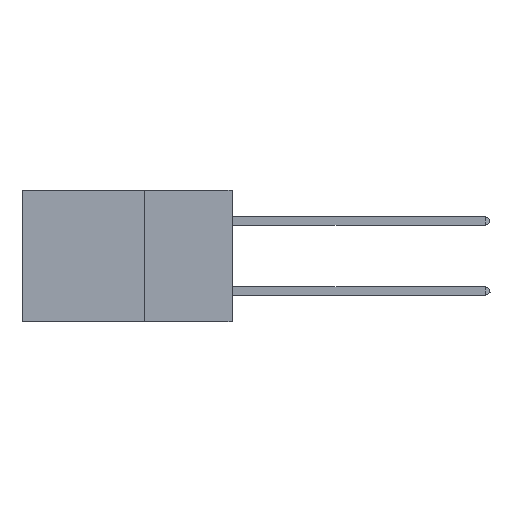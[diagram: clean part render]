
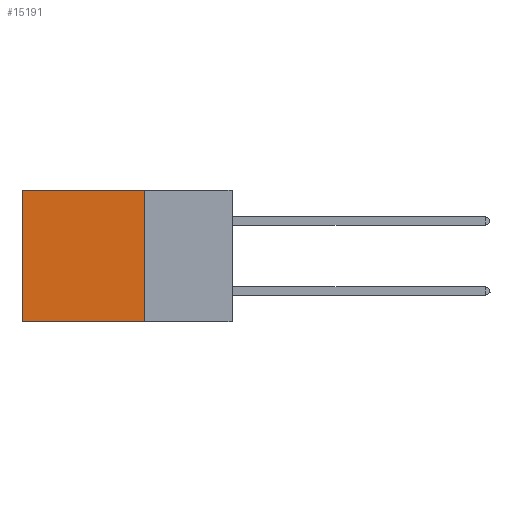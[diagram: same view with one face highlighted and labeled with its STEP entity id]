
A CAD part, left-side view. The second image highlights one B-rep face of the part: STEP entity #15191.
In plain terms, the highlighted planar face has unit normal (-1, 0, 0).
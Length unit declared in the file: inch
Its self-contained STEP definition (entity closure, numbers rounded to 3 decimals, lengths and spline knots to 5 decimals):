
#776 = CARTESIAN_POINT ( 'NONE',  ( 0.2875, 0.25, -0.375 ) ) ;
#837 = EDGE_CURVE ( 'NONE', #12370, #7916, #6039, .T. ) ;
#1363 = LINE ( 'NONE', #6219, #5033 ) ;
#2086 = VERTEX_POINT ( 'NONE', #9191 ) ;
#2201 = VERTEX_POINT ( 'NONE', #2952 ) ;
#2498 = DIRECTION ( 'NONE',  ( 0., 1., 0. ) ) ;
#2951 = AXIS2_PLACEMENT_3D ( 'NONE', #776, #13482, #11012 ) ;
#2952 = CARTESIAN_POINT ( 'NONE',  ( 0.2875, 0.25, -0.375 ) ) ;
#3482 = ORIENTED_EDGE ( 'NONE', *, *, #11682, .T. ) ;
#4158 = DIRECTION ( 'NONE',  ( 0., 1., 0. ) ) ;
#4168 = CARTESIAN_POINT ( 'NONE',  ( 0.2875, 0.25, 0. ) ) ;
#4285 = VECTOR ( 'NONE', #5078, 39.37008 ) ;
#4641 = EDGE_CURVE ( 'NONE', #12370, #2201, #6537, .T. ) ;
#5033 = VECTOR ( 'NONE', #2498, 39.37008 ) ;
#5072 = ORIENTED_EDGE ( 'NONE', *, *, #837, .T. ) ;
#5078 = DIRECTION ( 'NONE',  ( 0., 0., -1. ) ) ;
#6039 = LINE ( 'NONE', #11885, #15921 ) ;
#6219 = CARTESIAN_POINT ( 'NONE',  ( 0.2875, 0.25, -0.375 ) ) ;
#6537 = LINE ( 'NONE', #11353, #16398 ) ;
#6793 = CARTESIAN_POINT ( 'NONE',  ( 0.2875, 0.6, 0. ) ) ;
#7143 = EDGE_CURVE ( 'NONE', #2201, #2086, #1363, .T. ) ;
#7469 = CARTESIAN_POINT ( 'NONE',  ( 0.2875, 0.6, -0.375 ) ) ;
#7916 = VERTEX_POINT ( 'NONE', #6793 ) ;
#8166 = EDGE_LOOP ( 'NONE', ( #3482, #13172, #10596, #5072 ) ) ;
#8631 = DIRECTION ( 'NONE',  ( 0., 0., -1. ) ) ;
#9191 = CARTESIAN_POINT ( 'NONE',  ( 0.2875, 0.6, -0.375 ) ) ;
#10596 = ORIENTED_EDGE ( 'NONE', *, *, #4641, .F. ) ;
#10878 = FACE_OUTER_BOUND ( 'NONE', #8166, .T. ) ;
#11012 = DIRECTION ( 'NONE',  ( 0., 0., -1. ) ) ;
#11353 = CARTESIAN_POINT ( 'NONE',  ( 0.2875, 0.25, -0.375 ) ) ;
#11682 = EDGE_CURVE ( 'NONE', #7916, #2086, #14784, .T. ) ;
#11885 = CARTESIAN_POINT ( 'NONE',  ( 0.2875, 0.25, 0. ) ) ;
#12370 = VERTEX_POINT ( 'NONE', #4168 ) ;
#13172 = ORIENTED_EDGE ( 'NONE', *, *, #7143, .F. ) ;
#13482 = DIRECTION ( 'NONE',  ( 1., 0., 0. ) ) ;
#14784 = LINE ( 'NONE', #7469, #4285 ) ;
#15191 = ADVANCED_FACE ( 'NONE', ( #10878 ), #16084, .F. ) ;
#15921 = VECTOR ( 'NONE', #4158, 39.37008 ) ;
#16084 = PLANE ( 'NONE',  #2951 ) ;
#16398 = VECTOR ( 'NONE', #8631, 39.37008 ) ;
